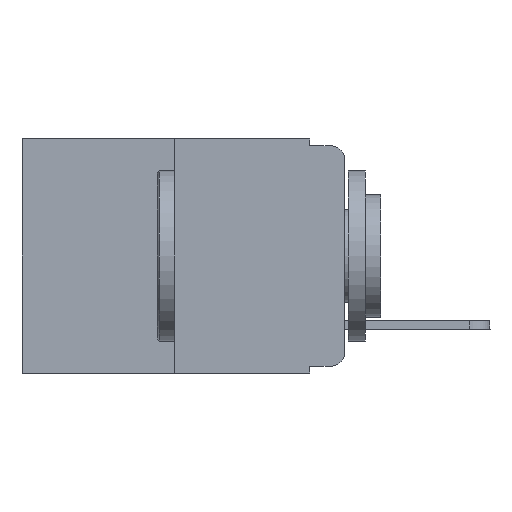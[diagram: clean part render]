
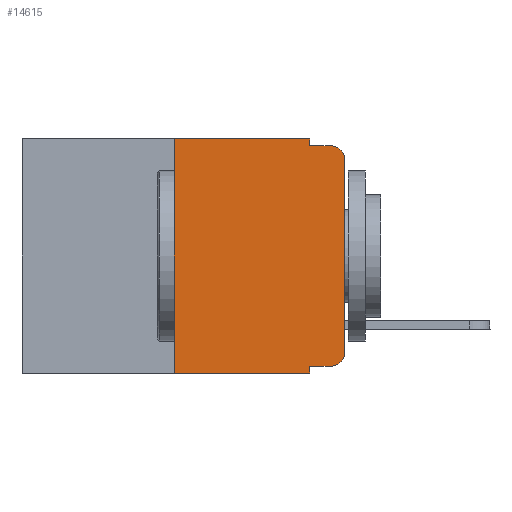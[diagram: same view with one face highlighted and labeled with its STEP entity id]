
A CAD part, left-side view. The second image highlights one B-rep face of the part: STEP entity #14615.
In plain terms, the highlighted planar face has unit normal (-1, 0, 0).
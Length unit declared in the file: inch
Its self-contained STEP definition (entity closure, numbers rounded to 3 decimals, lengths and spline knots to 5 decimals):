
#107 = VERTEX_POINT ( 'NONE', #13896 ) ;
#134 = ORIENTED_EDGE ( 'NONE', *, *, #11868, .T. ) ;
#189 = CARTESIAN_POINT ( 'NONE',  ( 0., 0.473, 0. ) ) ;
#399 = VERTEX_POINT ( 'NONE', #5750 ) ;
#431 = VERTEX_POINT ( 'NONE', #2228 ) ;
#514 = DIRECTION ( 'NONE',  ( -1., 0., 0. ) ) ;
#652 = VERTEX_POINT ( 'NONE', #14408 ) ;
#886 = DIRECTION ( 'NONE',  ( 0., -1., 0. ) ) ;
#956 = EDGE_CURVE ( 'NONE', #11573, #431, #3665, .T. ) ;
#1124 = CARTESIAN_POINT ( 'NONE',  ( 0., 0., 0. ) ) ;
#1126 = DIRECTION ( 'NONE',  ( 0., -1., 0. ) ) ;
#1149 = CARTESIAN_POINT ( 'NONE',  ( 0., 0.25, 0. ) ) ;
#1220 = DIRECTION ( 'NONE',  ( 0., -1., 0. ) ) ;
#1299 = EDGE_CURVE ( 'NONE', #652, #12448, #13900, .T. ) ;
#1505 = ORIENTED_EDGE ( 'NONE', *, *, #11240, .F. ) ;
#1660 = EDGE_CURVE ( 'NONE', #8340, #11800, #8996, .T. ) ;
#1677 = CIRCLE ( 'NONE', #8995, 0.02 ) ;
#1834 = ORIENTED_EDGE ( 'NONE', *, *, #2687, .T. ) ;
#2139 = CIRCLE ( 'NONE', #9955, 0.02 ) ;
#2228 = CARTESIAN_POINT ( 'NONE',  ( 0., 0.02, -0.01 ) ) ;
#2368 = LINE ( 'NONE', #1149, #7945 ) ;
#2687 = EDGE_CURVE ( 'NONE', #9192, #13700, #7018, .T. ) ;
#2824 = ORIENTED_EDGE ( 'NONE', *, *, #956, .F. ) ;
#2945 = DIRECTION ( 'NONE',  ( -1., 0., 0. ) ) ;
#3212 = VECTOR ( 'NONE', #4002, 39.37008 ) ;
#3644 = EDGE_CURVE ( 'NONE', #9192, #399, #8444, .T. ) ;
#3665 = LINE ( 'NONE', #10392, #10757 ) ;
#3717 = CARTESIAN_POINT ( 'NONE',  ( 0., 0.051, -0.333 ) ) ;
#3872 = VECTOR ( 'NONE', #10407, 39.37008 ) ;
#4002 = DIRECTION ( 'NONE',  ( 0., 0., -1. ) ) ;
#4014 = ORIENTED_EDGE ( 'NONE', *, *, #1660, .F. ) ;
#4191 = CARTESIAN_POINT ( 'NONE',  ( 0., 0.473, 0. ) ) ;
#4262 = VECTOR ( 'NONE', #7015, 39.37008 ) ;
#4682 = ORIENTED_EDGE ( 'NONE', *, *, #12685, .T. ) ;
#5159 = CARTESIAN_POINT ( 'NONE',  ( 0., 0.051, 0. ) ) ;
#5254 = CARTESIAN_POINT ( 'NONE',  ( 0., 0.051, 0. ) ) ;
#5750 = CARTESIAN_POINT ( 'NONE',  ( 0., 0.051, -0.343 ) ) ;
#6413 = EDGE_CURVE ( 'NONE', #107, #8340, #2368, .T. ) ;
#6661 = ORIENTED_EDGE ( 'NONE', *, *, #9404, .T. ) ;
#6879 = CARTESIAN_POINT ( 'NONE',  ( 0., 0.051, -0.333 ) ) ;
#6912 = CARTESIAN_POINT ( 'NONE',  ( 0., 0.02, -0.333 ) ) ;
#7015 = DIRECTION ( 'NONE',  ( 0., 0., 1. ) ) ;
#7018 = LINE ( 'NONE', #6879, #14817 ) ;
#7181 = ORIENTED_EDGE ( 'NONE', *, *, #3644, .F. ) ;
#7195 = DIRECTION ( 'NONE',  ( 0., 0., 1. ) ) ;
#7552 = DIRECTION ( 'NONE',  ( 0., 0., -1. ) ) ;
#7644 = CARTESIAN_POINT ( 'NONE',  ( 0., 0.473, -0.343 ) ) ;
#7945 = VECTOR ( 'NONE', #7195, 39.37008 ) ;
#8340 = VERTEX_POINT ( 'NONE', #14240 ) ;
#8384 = DIRECTION ( 'NONE',  ( 1., 0., 0. ) ) ;
#8444 = LINE ( 'NONE', #5159, #3212 ) ;
#8550 = EDGE_LOOP ( 'NONE', ( #11387, #134, #2824, #1505, #4014, #9552, #4682, #7181, #1834, #6661 ) ) ;
#8995 = AXIS2_PLACEMENT_3D ( 'NONE', #9759, #2945, #14436 ) ;
#8996 = LINE ( 'NONE', #4191, #13223 ) ;
#9192 = VERTEX_POINT ( 'NONE', #3717 ) ;
#9268 = LINE ( 'NONE', #13782, #3872 ) ;
#9358 = FACE_OUTER_BOUND ( 'NONE', #8550, .T. ) ;
#9404 = EDGE_CURVE ( 'NONE', #13700, #652, #2139, .T. ) ;
#9552 = ORIENTED_EDGE ( 'NONE', *, *, #6413, .F. ) ;
#9759 = CARTESIAN_POINT ( 'NONE',  ( 0., 0.02, -0.03 ) ) ;
#9804 = CARTESIAN_POINT ( 'NONE',  ( 0., 0.051, -0.01 ) ) ;
#9955 = AXIS2_PLACEMENT_3D ( 'NONE', #12198, #514, #7552 ) ;
#10387 = CARTESIAN_POINT ( 'NONE',  ( 0., 0., -0.03 ) ) ;
#10392 = CARTESIAN_POINT ( 'NONE',  ( 0., 0.051, -0.01 ) ) ;
#10407 = DIRECTION ( 'NONE',  ( 0., 0., -1. ) ) ;
#10757 = VECTOR ( 'NONE', #1220, 39.37008 ) ;
#11240 = EDGE_CURVE ( 'NONE', #11800, #11573, #9268, .T. ) ;
#11387 = ORIENTED_EDGE ( 'NONE', *, *, #1299, .T. ) ;
#11573 = VERTEX_POINT ( 'NONE', #9804 ) ;
#11800 = VERTEX_POINT ( 'NONE', #5254 ) ;
#11868 = EDGE_CURVE ( 'NONE', #12448, #431, #1677, .T. ) ;
#12072 = LINE ( 'NONE', #7644, #14413 ) ;
#12198 = CARTESIAN_POINT ( 'NONE',  ( 0., 0.02, -0.313 ) ) ;
#12242 = AXIS2_PLACEMENT_3D ( 'NONE', #189, #8384, #13040 ) ;
#12448 = VERTEX_POINT ( 'NONE', #10387 ) ;
#12685 = EDGE_CURVE ( 'NONE', #107, #399, #12072, .T. ) ;
#13040 = DIRECTION ( 'NONE',  ( 0., 0., -1. ) ) ;
#13223 = VECTOR ( 'NONE', #886, 39.37008 ) ;
#13700 = VERTEX_POINT ( 'NONE', #6912 ) ;
#13782 = CARTESIAN_POINT ( 'NONE',  ( 0., 0.051, 0. ) ) ;
#13896 = CARTESIAN_POINT ( 'NONE',  ( 0., 0.25, -0.343 ) ) ;
#13900 = LINE ( 'NONE', #1124, #4262 ) ;
#14043 = PLANE ( 'NONE',  #12242 ) ;
#14240 = CARTESIAN_POINT ( 'NONE',  ( 0., 0.25, 0. ) ) ;
#14408 = CARTESIAN_POINT ( 'NONE',  ( 0., 0., -0.313 ) ) ;
#14413 = VECTOR ( 'NONE', #14675, 39.37008 ) ;
#14436 = DIRECTION ( 'NONE',  ( 0., 0., -1. ) ) ;
#14615 = ADVANCED_FACE ( 'NONE', ( #9358 ), #14043, .F. ) ;
#14675 = DIRECTION ( 'NONE',  ( 0., -1., 0. ) ) ;
#14817 = VECTOR ( 'NONE', #1126, 39.37008 ) ;
